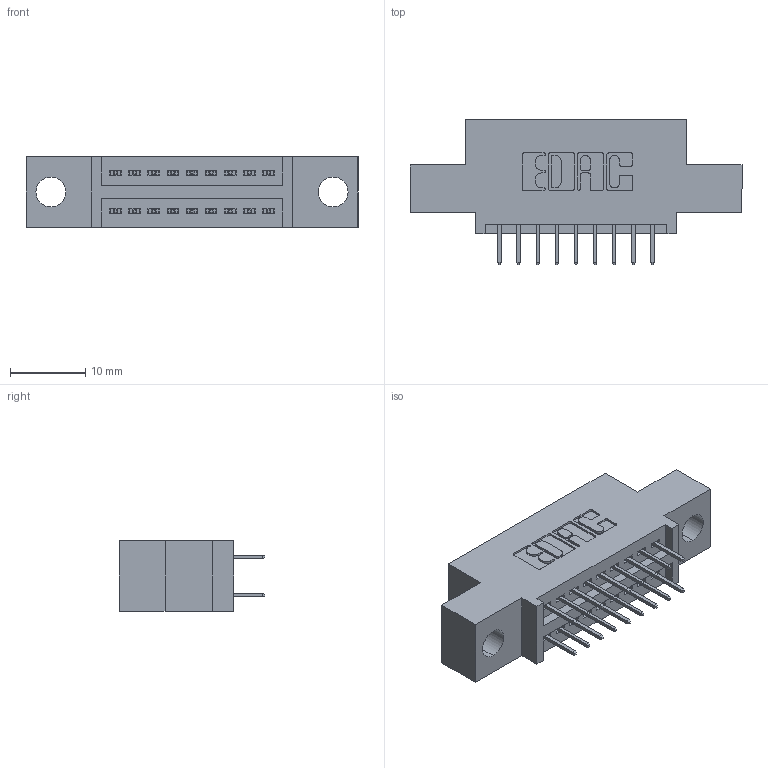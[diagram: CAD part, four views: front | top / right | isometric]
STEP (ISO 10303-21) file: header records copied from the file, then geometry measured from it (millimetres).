
FILE_DESCRIPTION (( 'STEP AP203' ), '1' );
FILE_NAME ('345-018-524-504.STEP', '2018-08-19T07:08:30', ( '' ), ( '' ), 'SwSTEP 2.0', 'SolidWorks 2016', '' );
FILE_SCHEMA (( 'CONFIG_CONTROL_DESIGN' ));
Length unit declared in the file: inch
Products named in the file (3): 345 Part_0.110 Offset - 0.156 Dia-TH; 345-292-001_345-293-124; 345-018-524-504
Assembly tree (19 placements, depth 2):
  345-018-524-504
    345 Part_0.110 Offset - 0.156 Dia-TH
    345-292-001_345-293-124  x18
Bounding box: 44.07 x 19.35 x 9.4 mm (x, y, z)
Volume: 3786.1 mm3; surface area: 4793.5 mm2
Topology: 19 solids, 19 shells, 1102 faces, 3107 edges, 1998 vertices
Faces by surface type: plane 786, cylinder 316
Entity records: 11713 total; most frequent: CARTESIAN_POINT 1996, ORIENTED_EDGE 1930, DIRECTION 1801, EDGE_CURVE 965, LINE 801, VECTOR 801, VERTEX_POINT 638, AXIS2_PLACEMENT_3D 500
